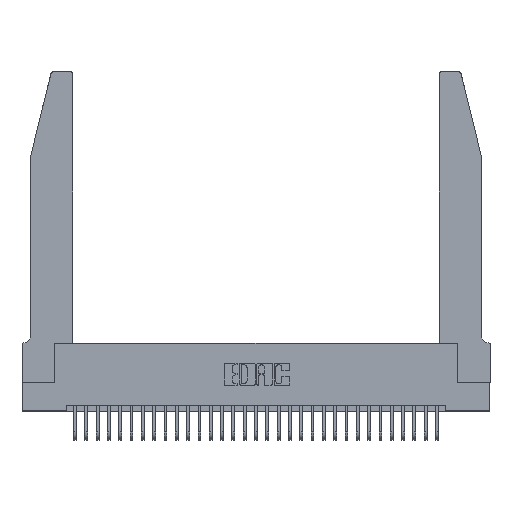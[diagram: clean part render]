
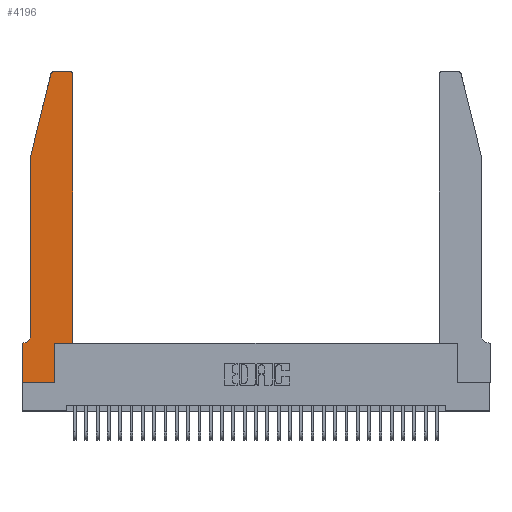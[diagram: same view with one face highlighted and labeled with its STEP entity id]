
A CAD part, top view. The second image highlights one B-rep face of the part: STEP entity #4196.
In plain terms, the highlighted planar face has unit normal (0, 0, 1).
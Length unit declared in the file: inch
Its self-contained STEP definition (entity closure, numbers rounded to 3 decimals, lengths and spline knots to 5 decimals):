
#146 = DIRECTION ( 'NONE',  ( -1., 0., 0. ) ) ;
#465 = LINE ( 'NONE', #31900, #6700 ) ;
#737 = EDGE_CURVE ( 'NONE', #1193, #13938, #28326, .T. ) ;
#862 = VERTEX_POINT ( 'NONE', #11958 ) ;
#1147 = LINE ( 'NONE', #15184, #27959 ) ;
#1193 = VERTEX_POINT ( 'NONE', #11918 ) ;
#1224 = DIRECTION ( 'NONE',  ( 1., 0., 0. ) ) ;
#1244 = AXIS2_PLACEMENT_3D ( 'NONE', #10339, #28339, #12922 ) ;
#2529 = EDGE_LOOP ( 'NONE', ( #26443, #30952, #29176, #8448, #21302, #22081, #8151, #15193, #17463, #17666, #27153, #8128 ) ) ;
#3419 = CARTESIAN_POINT ( 'NONE',  ( 0.4205, 2.75, 0.37 ) ) ;
#3470 = VERTEX_POINT ( 'NONE', #3419 ) ;
#3651 = VERTEX_POINT ( 'NONE', #30116 ) ;
#4196 = ADVANCED_FACE ( 'NONE', ( #19206 ), #18424, .T. ) ;
#5212 = DIRECTION ( 'NONE',  ( -0.239, -0.971, 0. ) ) ;
#5213 = CARTESIAN_POINT ( 'NONE',  ( 0.4505, 2.72, 0.37 ) ) ;
#5512 = AXIS2_PLACEMENT_3D ( 'NONE', #15238, #33202, #17835 ) ;
#6442 = CARTESIAN_POINT ( 'NONE',  ( 0.0755, 2., 0.37 ) ) ;
#6700 = VECTOR ( 'NONE', #11350, 39.37008 ) ;
#7292 = EDGE_CURVE ( 'NONE', #8057, #16031, #17156, .T. ) ;
#7602 = LINE ( 'NONE', #21101, #28164 ) ;
#7664 = VERTEX_POINT ( 'NONE', #23064 ) ;
#7866 = CARTESIAN_POINT ( 'NONE',  ( 0.0755, 2., 0.37 ) ) ;
#8057 = VERTEX_POINT ( 'NONE', #8922 ) ;
#8128 = ORIENTED_EDGE ( 'NONE', *, *, #32198, .T. ) ;
#8151 = ORIENTED_EDGE ( 'NONE', *, *, #26852, .T. ) ;
#8259 = EDGE_CURVE ( 'NONE', #13938, #22988, #15475, .T. ) ;
#8448 = ORIENTED_EDGE ( 'NONE', *, *, #18202, .T. ) ;
#8483 = EDGE_CURVE ( 'NONE', #3651, #862, #10655, .T. ) ;
#8922 = CARTESIAN_POINT ( 'NONE',  ( 0.0055, 0.35, 0.37 ) ) ;
#9073 = DIRECTION ( 'NONE',  ( 0., -1., 0. ) ) ;
#9516 = VECTOR ( 'NONE', #16411, 39.37008 ) ;
#9586 = CARTESIAN_POINT ( 'NONE',  ( 0.4505, 0.35, 0.37 ) ) ;
#10267 = VECTOR ( 'NONE', #25153, 39.37008 ) ;
#10339 = CARTESIAN_POINT ( 'NONE',  ( 0.284, 2.72, 0.37 ) ) ;
#10627 = DIRECTION ( 'NONE',  ( 1., 0., 0. ) ) ;
#10655 = LINE ( 'NONE', #28617, #15865 ) ;
#10793 = DIRECTION ( 'NONE',  ( 1., 0., 0. ) ) ;
#10870 = EDGE_CURVE ( 'NONE', #7664, #8057, #21403, .T. ) ;
#11350 = DIRECTION ( 'NONE',  ( -1., 0., 0. ) ) ;
#11632 = CARTESIAN_POINT ( 'NONE',  ( 0.25487, 2.72718, 0.37 ) ) ;
#11689 = EDGE_CURVE ( 'NONE', #3470, #14024, #465, .T. ) ;
#11918 = CARTESIAN_POINT ( 'NONE',  ( 0.2865, 0.35, 0.37 ) ) ;
#11958 = CARTESIAN_POINT ( 'NONE',  ( 0.2865, 0., 0.37 ) ) ;
#12922 = DIRECTION ( 'NONE',  ( 1., 0., 0. ) ) ;
#13392 = CARTESIAN_POINT ( 'NONE',  ( 0.284, 2.75, 0.37 ) ) ;
#13938 = VERTEX_POINT ( 'NONE', #20831 ) ;
#14024 = VERTEX_POINT ( 'NONE', #13392 ) ;
#15184 = CARTESIAN_POINT ( 'NONE',  ( 0., 0., 0.37 ) ) ;
#15193 = ORIENTED_EDGE ( 'NONE', *, *, #8483, .T. ) ;
#15238 = CARTESIAN_POINT ( 'NONE',  ( 0.4205, 2.72, 0.37 ) ) ;
#15259 = CIRCLE ( 'NONE', #1244, 0.03 ) ;
#15475 = LINE ( 'NONE', #25051, #10267 ) ;
#15804 = DIRECTION ( 'NONE',  ( 0., 0., -1. ) ) ;
#15865 = VECTOR ( 'NONE', #10627, 39.37008 ) ;
#16031 = VERTEX_POINT ( 'NONE', #20706 ) ;
#16411 = DIRECTION ( 'NONE',  ( -1., 0., 0. ) ) ;
#17156 = LINE ( 'NONE', #21585, #9516 ) ;
#17321 = EDGE_CURVE ( 'NONE', #24379, #18429, #24958, .T. ) ;
#17463 = ORIENTED_EDGE ( 'NONE', *, *, #20985, .T. ) ;
#17666 = ORIENTED_EDGE ( 'NONE', *, *, #737, .T. ) ;
#17835 = DIRECTION ( 'NONE',  ( 1., 0., 0. ) ) ;
#18101 = VECTOR ( 'NONE', #5212, 39.37008 ) ;
#18202 = EDGE_CURVE ( 'NONE', #18429, #7664, #29150, .T. ) ;
#18424 = PLANE ( 'NONE',  #25242 ) ;
#18429 = VERTEX_POINT ( 'NONE', #23636 ) ;
#19206 = FACE_OUTER_BOUND ( 'NONE', #2529, .T. ) ;
#20290 = CIRCLE ( 'NONE', #5512, 0.03 ) ;
#20706 = CARTESIAN_POINT ( 'NONE',  ( 0., 0.35, 0.37 ) ) ;
#20831 = CARTESIAN_POINT ( 'NONE',  ( 0.4505, 0.35, 0.37 ) ) ;
#20985 = EDGE_CURVE ( 'NONE', #862, #1193, #7602, .T. ) ;
#21101 = CARTESIAN_POINT ( 'NONE',  ( 0.2865, 0.35, 0.37 ) ) ;
#21302 = ORIENTED_EDGE ( 'NONE', *, *, #10870, .T. ) ;
#21403 = CIRCLE ( 'NONE', #24967, 0.07 ) ;
#21472 = VECTOR ( 'NONE', #1224, 39.37008 ) ;
#21585 = CARTESIAN_POINT ( 'NONE',  ( 0.0755, 0.35, 0.37 ) ) ;
#22081 = ORIENTED_EDGE ( 'NONE', *, *, #7292, .T. ) ;
#22988 = VERTEX_POINT ( 'NONE', #5213 ) ;
#23064 = CARTESIAN_POINT ( 'NONE',  ( 0.0755, 0.42, 0.37 ) ) ;
#23623 = CARTESIAN_POINT ( 'NONE',  ( 0., 0.35, 0.37 ) ) ;
#23636 = CARTESIAN_POINT ( 'NONE',  ( 0.0755, 2., 0.37 ) ) ;
#23695 = DIRECTION ( 'NONE',  ( 0., 1., 0. ) ) ;
#24379 = VERTEX_POINT ( 'NONE', #11632 ) ;
#24958 = LINE ( 'NONE', #7866, #18101 ) ;
#24967 = AXIS2_PLACEMENT_3D ( 'NONE', #31176, #15804, #146 ) ;
#25051 = CARTESIAN_POINT ( 'NONE',  ( 0.4505, 0.35, 0.37 ) ) ;
#25153 = DIRECTION ( 'NONE',  ( 0., 1., 0. ) ) ;
#25242 = AXIS2_PLACEMENT_3D ( 'NONE', #23623, #26224, #10793 ) ;
#26224 = DIRECTION ( 'NONE',  ( 0., 0., 1. ) ) ;
#26443 = ORIENTED_EDGE ( 'NONE', *, *, #11689, .T. ) ;
#26852 = EDGE_CURVE ( 'NONE', #16031, #3651, #1147, .T. ) ;
#27153 = ORIENTED_EDGE ( 'NONE', *, *, #8259, .T. ) ;
#27959 = VECTOR ( 'NONE', #30599, 39.37008 ) ;
#28164 = VECTOR ( 'NONE', #23695, 39.37008 ) ;
#28326 = LINE ( 'NONE', #9586, #21472 ) ;
#28339 = DIRECTION ( 'NONE',  ( 0., 0., 1. ) ) ;
#28354 = VECTOR ( 'NONE', #9073, 39.37008 ) ;
#28617 = CARTESIAN_POINT ( 'NONE',  ( 0., 0., 0.37 ) ) ;
#29150 = LINE ( 'NONE', #6442, #28354 ) ;
#29176 = ORIENTED_EDGE ( 'NONE', *, *, #17321, .T. ) ;
#29775 = EDGE_CURVE ( 'NONE', #14024, #24379, #15259, .T. ) ;
#30116 = CARTESIAN_POINT ( 'NONE',  ( 0., 0., 0.37 ) ) ;
#30599 = DIRECTION ( 'NONE',  ( 0., -1., 0. ) ) ;
#30952 = ORIENTED_EDGE ( 'NONE', *, *, #29775, .T. ) ;
#31176 = CARTESIAN_POINT ( 'NONE',  ( 0.0055, 0.42, 0.37 ) ) ;
#31900 = CARTESIAN_POINT ( 'NONE',  ( 0.2605, 2.75, 0.37 ) ) ;
#32198 = EDGE_CURVE ( 'NONE', #22988, #3470, #20290, .T. ) ;
#33202 = DIRECTION ( 'NONE',  ( 0., 0., 1. ) ) ;
